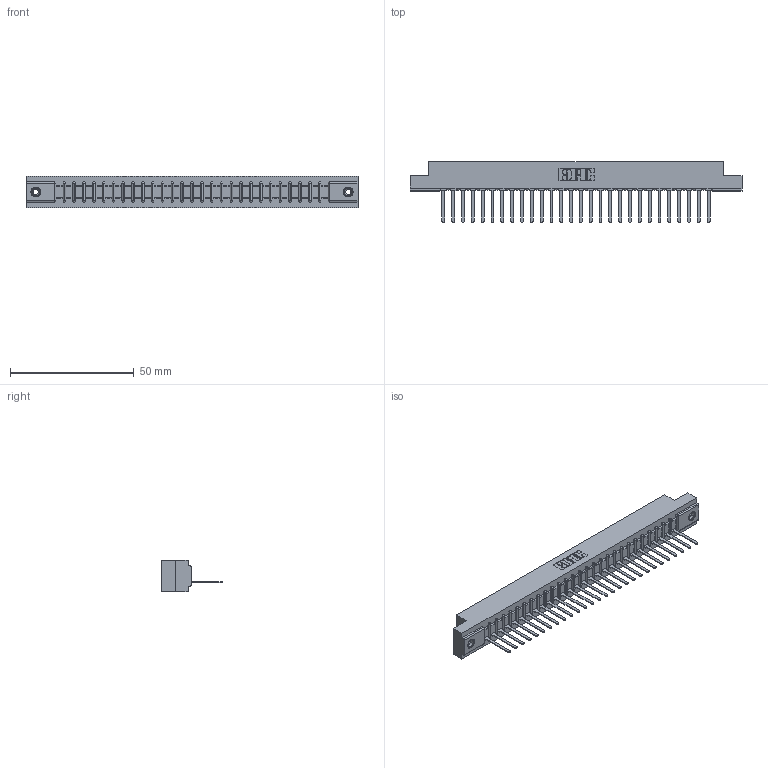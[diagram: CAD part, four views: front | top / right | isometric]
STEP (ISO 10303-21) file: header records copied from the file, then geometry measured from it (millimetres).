
FILE_DESCRIPTION (( 'STEP AP203' ), '1' );
FILE_NAME ('357-028-541-108.STEP', '2019-09-17T02:08:32', ( '' ), ( '' ), 'SwSTEP 2.0', 'SolidWorks 2016', '' );
FILE_SCHEMA (( 'CONFIG_CONTROL_DESIGN' ));
Length unit declared in the file: inch
Products named in the file (4): 307-290-002_541; 357-028-541-108; 307 Part_.156 Dia Mounting Holes; 345-250-001_345-250-003-102
Assembly tree (31 placements, depth 2):
  357-028-541-108
    307 Part_.156 Dia Mounting Holes
    307-290-002_541  x28
    345-250-001_345-250-003-102  x2
Bounding box: 133.96 x 24.59 x 12.7 mm (x, y, z)
Volume: 14303.5 mm3; surface area: 18206.3 mm2
Topology: 31 solids, 31 shells, 2279 faces, 6955 edges, 4550 vertices
Faces by surface type: plane 1362, cylinder 843, sphere 58, cone 12, torus 4
Entity records: 27633 total; most frequent: CARTESIAN_POINT 4639, ORIENTED_EDGE 4622, DIRECTION 4523, EDGE_CURVE 2311, VECTOR 1763, LINE 1763, VERTEX_POINT 1496, AXIS2_PLACEMENT_3D 1380
